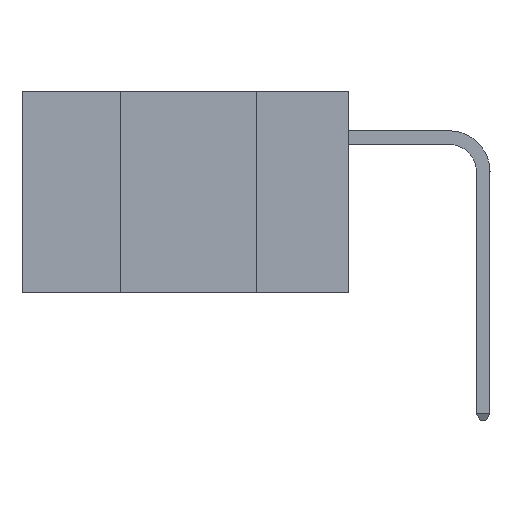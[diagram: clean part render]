
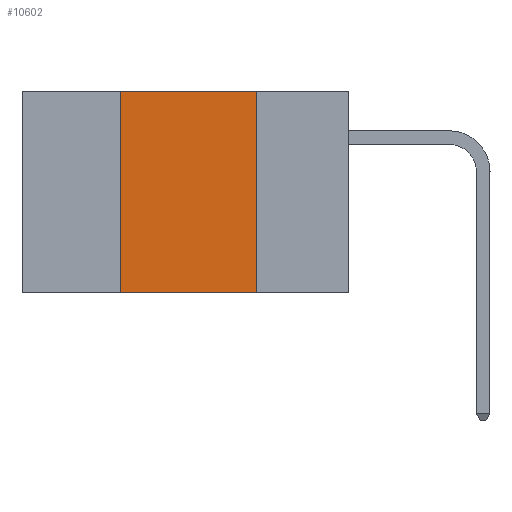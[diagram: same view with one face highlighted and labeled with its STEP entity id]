
A CAD part, left-side view. The second image highlights one B-rep face of the part: STEP entity #10602.
In plain terms, the highlighted planar face has unit normal (-1, 0, 0).
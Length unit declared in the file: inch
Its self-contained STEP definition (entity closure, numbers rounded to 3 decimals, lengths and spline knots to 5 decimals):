
#22 = VERTEX_POINT ( 'NONE', #6803 ) ;
#60 = CARTESIAN_POINT ( 'NONE',  ( 0., 0.6, -0.37 ) ) ;
#231 = EDGE_CURVE ( 'NONE', #22, #11180, #7458, .T. ) ;
#513 = CARTESIAN_POINT ( 'NONE',  ( 0., 0.6, 0. ) ) ;
#523 = EDGE_CURVE ( 'NONE', #4408, #569, #6026, .T. ) ;
#569 = VERTEX_POINT ( 'NONE', #1565 ) ;
#1302 = EDGE_CURVE ( 'NONE', #4408, #11180, #2209, .T. ) ;
#1320 = CARTESIAN_POINT ( 'NONE',  ( 0., 0.17, -0.37 ) ) ;
#1565 = CARTESIAN_POINT ( 'NONE',  ( 0., 0.42, 0. ) ) ;
#2209 = LINE ( 'NONE', #60, #8944 ) ;
#2304 = DIRECTION ( 'NONE',  ( 0., 0., 1. ) ) ;
#2333 = CARTESIAN_POINT ( 'NONE',  ( 0., 0.42, 0. ) ) ;
#2420 = EDGE_LOOP ( 'NONE', ( #9651, #3393, #10715, #6301 ) ) ;
#2534 = PLANE ( 'NONE',  #8555 ) ;
#3339 = LINE ( 'NONE', #9839, #7714 ) ;
#3393 = ORIENTED_EDGE ( 'NONE', *, *, #4224, .F. ) ;
#3582 = DIRECTION ( 'NONE',  ( 1., 0., 0. ) ) ;
#4224 = EDGE_CURVE ( 'NONE', #569, #22, #3339, .T. ) ;
#4408 = VERTEX_POINT ( 'NONE', #8586 ) ;
#5292 = DIRECTION ( 'NONE',  ( 0., 0., -1. ) ) ;
#5465 = CARTESIAN_POINT ( 'NONE',  ( 0., 0.17, 0. ) ) ;
#6026 = LINE ( 'NONE', #2333, #8695 ) ;
#6301 = ORIENTED_EDGE ( 'NONE', *, *, #1302, .T. ) ;
#6372 = DIRECTION ( 'NONE',  ( 0., -1., 0. ) ) ;
#6803 = CARTESIAN_POINT ( 'NONE',  ( 0., 0.17, 0. ) ) ;
#7458 = LINE ( 'NONE', #5465, #7728 ) ;
#7714 = VECTOR ( 'NONE', #9781, 39.37008 ) ;
#7728 = VECTOR ( 'NONE', #5292, 39.37008 ) ;
#8212 = FACE_OUTER_BOUND ( 'NONE', #2420, .T. ) ;
#8555 = AXIS2_PLACEMENT_3D ( 'NONE', #513, #3582, #9480 ) ;
#8586 = CARTESIAN_POINT ( 'NONE',  ( 0., 0.42, -0.37 ) ) ;
#8695 = VECTOR ( 'NONE', #2304, 39.37008 ) ;
#8944 = VECTOR ( 'NONE', #6372, 39.37008 ) ;
#9480 = DIRECTION ( 'NONE',  ( 0., 0., -1. ) ) ;
#9651 = ORIENTED_EDGE ( 'NONE', *, *, #231, .F. ) ;
#9781 = DIRECTION ( 'NONE',  ( 0., -1., 0. ) ) ;
#9839 = CARTESIAN_POINT ( 'NONE',  ( 0., 0.6, 0. ) ) ;
#10602 = ADVANCED_FACE ( 'NONE', ( #8212 ), #2534, .F. ) ;
#10715 = ORIENTED_EDGE ( 'NONE', *, *, #523, .F. ) ;
#11180 = VERTEX_POINT ( 'NONE', #1320 ) ;
